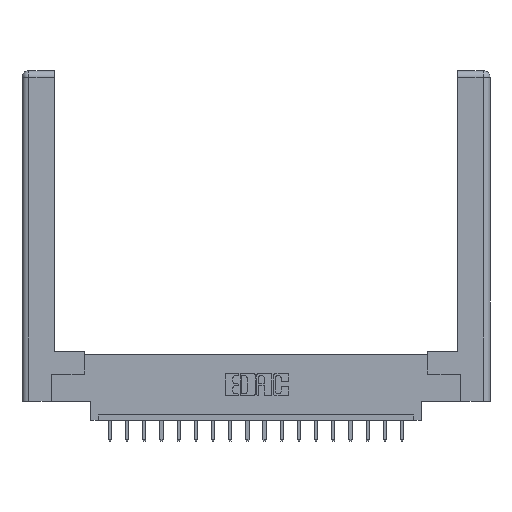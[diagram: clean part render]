
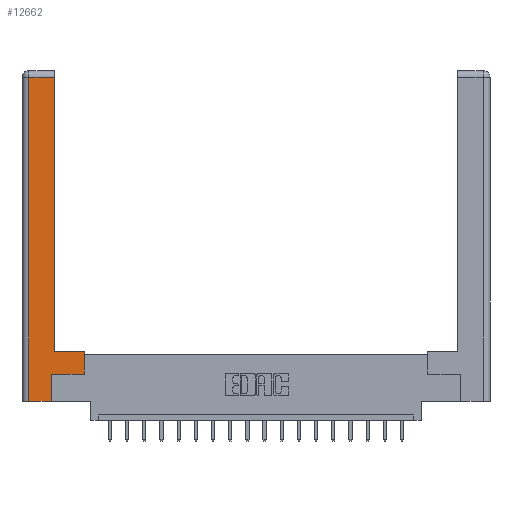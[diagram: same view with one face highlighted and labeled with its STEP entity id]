
A CAD part, top view. The second image highlights one B-rep face of the part: STEP entity #12662.
In plain terms, the highlighted planar face has unit normal (0, 0, 1).
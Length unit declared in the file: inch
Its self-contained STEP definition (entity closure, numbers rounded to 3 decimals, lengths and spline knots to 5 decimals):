
#79 = VECTOR ( 'NONE', #3877, 39.37008 ) ;
#550 = CARTESIAN_POINT ( 'NONE',  ( 0.565, 0.245, 0. ) ) ;
#646 = PLANE ( 'NONE',  #7333 ) ;
#712 = CARTESIAN_POINT ( 'NONE',  ( 0., 0., 0. ) ) ;
#727 = ORIENTED_EDGE ( 'NONE', *, *, #4262, .T. ) ;
#877 = EDGE_CURVE ( 'NONE', #13929, #9469, #15056, .T. ) ;
#881 = CARTESIAN_POINT ( 'NONE',  ( 0.265, 0., 0. ) ) ;
#1145 = DIRECTION ( 'NONE',  ( 1., 0., 0. ) ) ;
#1261 = CARTESIAN_POINT ( 'NONE',  ( 0.0615, 2.94, 0. ) ) ;
#1295 = LINE ( 'NONE', #13404, #16752 ) ;
#1874 = ORIENTED_EDGE ( 'NONE', *, *, #3995, .T. ) ;
#2542 = ORIENTED_EDGE ( 'NONE', *, *, #5259, .T. ) ;
#2651 = VECTOR ( 'NONE', #15296, 39.37008 ) ;
#2938 = CARTESIAN_POINT ( 'NONE',  ( 0.565, 0.45, 0. ) ) ;
#3009 = DIRECTION ( 'NONE',  ( 0., -1., 0. ) ) ;
#3770 = LINE ( 'NONE', #881, #9411 ) ;
#3773 = VERTEX_POINT ( 'NONE', #7611 ) ;
#3877 = DIRECTION ( 'NONE',  ( 0., 1., 0. ) ) ;
#3995 = EDGE_CURVE ( 'NONE', #9469, #3773, #12473, .T. ) ;
#4162 = VERTEX_POINT ( 'NONE', #6151 ) ;
#4262 = EDGE_CURVE ( 'NONE', #3773, #18008, #9214, .T. ) ;
#4505 = VERTEX_POINT ( 'NONE', #7250 ) ;
#4541 = VECTOR ( 'NONE', #11775, 39.37008 ) ;
#4901 = LINE ( 'NONE', #10262, #14251 ) ;
#5027 = LINE ( 'NONE', #18702, #79 ) ;
#5259 = EDGE_CURVE ( 'NONE', #4162, #16258, #3770, .T. ) ;
#6151 = CARTESIAN_POINT ( 'NONE',  ( 0.0615, 0., 0. ) ) ;
#6351 = CARTESIAN_POINT ( 'NONE',  ( 0.265, 0., 0. ) ) ;
#6574 = VECTOR ( 'NONE', #13065, 39.37008 ) ;
#7250 = CARTESIAN_POINT ( 'NONE',  ( 0.295, 2.94, 0. ) ) ;
#7308 = VERTEX_POINT ( 'NONE', #1261 ) ;
#7333 = AXIS2_PLACEMENT_3D ( 'NONE', #712, #15725, #9921 ) ;
#7523 = EDGE_CURVE ( 'NONE', #18008, #4505, #5027, .T. ) ;
#7611 = CARTESIAN_POINT ( 'NONE',  ( 0.565, 0.45, 0. ) ) ;
#7882 = CARTESIAN_POINT ( 'NONE',  ( 0.295, 0.45, 0. ) ) ;
#8109 = FACE_OUTER_BOUND ( 'NONE', #18650, .T. ) ;
#9214 = LINE ( 'NONE', #9636, #16456 ) ;
#9411 = VECTOR ( 'NONE', #1145, 39.37008 ) ;
#9469 = VERTEX_POINT ( 'NONE', #9851 ) ;
#9636 = CARTESIAN_POINT ( 'NONE',  ( 0.295, 0.45, 0. ) ) ;
#9851 = CARTESIAN_POINT ( 'NONE',  ( 0.565, 0.245, 0. ) ) ;
#9871 = EDGE_CURVE ( 'NONE', #16258, #13929, #18502, .T. ) ;
#9921 = DIRECTION ( 'NONE',  ( -1., 0., 0. ) ) ;
#10262 = CARTESIAN_POINT ( 'NONE',  ( 0.0615, 2.94, 0. ) ) ;
#11335 = CARTESIAN_POINT ( 'NONE',  ( 0.265, 0.245, 0. ) ) ;
#11775 = DIRECTION ( 'NONE',  ( 0., 1., 0. ) ) ;
#12473 = LINE ( 'NONE', #2938, #4541 ) ;
#12662 = ADVANCED_FACE ( 'NONE', ( #8109 ), #646, .F. ) ;
#13065 = DIRECTION ( 'NONE',  ( 0., 1., 0. ) ) ;
#13404 = CARTESIAN_POINT ( 'NONE',  ( 0.0615, 0., 0. ) ) ;
#13924 = EDGE_CURVE ( 'NONE', #4505, #7308, #4901, .T. ) ;
#13929 = VERTEX_POINT ( 'NONE', #16214 ) ;
#13989 = DIRECTION ( 'NONE',  ( -1., 0., 0. ) ) ;
#14251 = VECTOR ( 'NONE', #19062, 39.37008 ) ;
#15056 = LINE ( 'NONE', #550, #2651 ) ;
#15296 = DIRECTION ( 'NONE',  ( 1., 0., 0. ) ) ;
#15656 = ORIENTED_EDGE ( 'NONE', *, *, #13924, .T. ) ;
#15671 = EDGE_CURVE ( 'NONE', #7308, #4162, #1295, .T. ) ;
#15725 = DIRECTION ( 'NONE',  ( 0., 0., -1. ) ) ;
#16214 = CARTESIAN_POINT ( 'NONE',  ( 0.265, 0.245, 0. ) ) ;
#16258 = VERTEX_POINT ( 'NONE', #6351 ) ;
#16456 = VECTOR ( 'NONE', #13989, 39.37008 ) ;
#16752 = VECTOR ( 'NONE', #3009, 39.37008 ) ;
#16770 = ORIENTED_EDGE ( 'NONE', *, *, #15671, .T. ) ;
#17267 = ORIENTED_EDGE ( 'NONE', *, *, #877, .T. ) ;
#18008 = VERTEX_POINT ( 'NONE', #7882 ) ;
#18502 = LINE ( 'NONE', #11335, #6574 ) ;
#18633 = ORIENTED_EDGE ( 'NONE', *, *, #7523, .T. ) ;
#18650 = EDGE_LOOP ( 'NONE', ( #18633, #15656, #16770, #2542, #18984, #17267, #1874, #727 ) ) ;
#18702 = CARTESIAN_POINT ( 'NONE',  ( 0.295, 3., 0. ) ) ;
#18984 = ORIENTED_EDGE ( 'NONE', *, *, #9871, .T. ) ;
#19062 = DIRECTION ( 'NONE',  ( -1., 0., 0. ) ) ;
